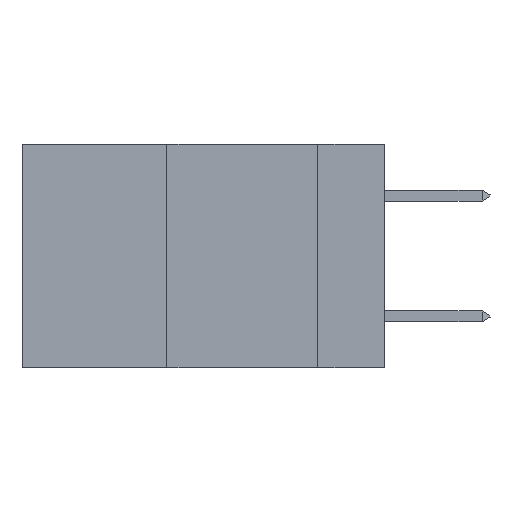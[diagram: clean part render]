
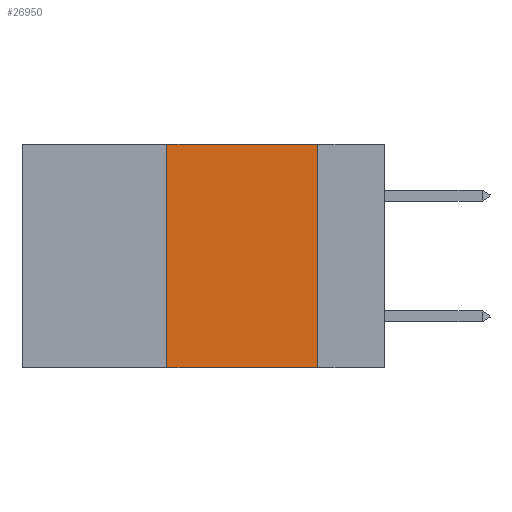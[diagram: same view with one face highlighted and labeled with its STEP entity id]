
A CAD part, left-side view. The second image highlights one B-rep face of the part: STEP entity #26950.
In plain terms, the highlighted planar face has unit normal (-1, 0, 0).
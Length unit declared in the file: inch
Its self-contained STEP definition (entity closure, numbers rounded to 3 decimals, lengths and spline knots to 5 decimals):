
#184 = VECTOR ( 'NONE', #4206, 39.37008 ) ;
#1067 = DIRECTION ( 'NONE',  ( 0., 0., -1. ) ) ;
#1257 = CARTESIAN_POINT ( 'NONE',  ( 0., 0.11, -0.37 ) ) ;
#2582 = CARTESIAN_POINT ( 'NONE',  ( 0., 0.6, -0.37 ) ) ;
#2880 = EDGE_LOOP ( 'NONE', ( #27715, #11392, #15418, #25714 ) ) ;
#3241 = CARTESIAN_POINT ( 'NONE',  ( 0., 0.6, 0. ) ) ;
#4206 = DIRECTION ( 'NONE',  ( 0., 0., 1. ) ) ;
#5151 = CARTESIAN_POINT ( 'NONE',  ( 0., 0.6, 0. ) ) ;
#6396 = VECTOR ( 'NONE', #27326, 39.37008 ) ;
#6772 = AXIS2_PLACEMENT_3D ( 'NONE', #3241, #17424, #1067 ) ;
#6932 = EDGE_CURVE ( 'NONE', #11074, #27075, #13192, .T. ) ;
#7243 = LINE ( 'NONE', #22990, #184 ) ;
#7800 = LINE ( 'NONE', #2582, #27742 ) ;
#9862 = VECTOR ( 'NONE', #24137, 39.37008 ) ;
#10455 = PLANE ( 'NONE',  #6772 ) ;
#10958 = CARTESIAN_POINT ( 'NONE',  ( 0., 0.11, 0. ) ) ;
#11074 = VERTEX_POINT ( 'NONE', #20526 ) ;
#11392 = ORIENTED_EDGE ( 'NONE', *, *, #6932, .F. ) ;
#12003 = EDGE_CURVE ( 'NONE', #27075, #12298, #18589, .T. ) ;
#12298 = VERTEX_POINT ( 'NONE', #1257 ) ;
#13192 = LINE ( 'NONE', #5151, #9862 ) ;
#15418 = ORIENTED_EDGE ( 'NONE', *, *, #27625, .F. ) ;
#17424 = DIRECTION ( 'NONE',  ( 1., 0., 0. ) ) ;
#17746 = CARTESIAN_POINT ( 'NONE',  ( 0., 0.11, 0. ) ) ;
#18307 = EDGE_CURVE ( 'NONE', #19309, #12298, #7800, .T. ) ;
#18589 = LINE ( 'NONE', #17746, #6396 ) ;
#19309 = VERTEX_POINT ( 'NONE', #25173 ) ;
#20526 = CARTESIAN_POINT ( 'NONE',  ( 0., 0.36, 0. ) ) ;
#22990 = CARTESIAN_POINT ( 'NONE',  ( 0., 0.36, 0. ) ) ;
#24137 = DIRECTION ( 'NONE',  ( 0., -1., 0. ) ) ;
#25173 = CARTESIAN_POINT ( 'NONE',  ( 0., 0.36, -0.37 ) ) ;
#25714 = ORIENTED_EDGE ( 'NONE', *, *, #18307, .T. ) ;
#26950 = ADVANCED_FACE ( 'NONE', ( #28000 ), #10455, .F. ) ;
#27075 = VERTEX_POINT ( 'NONE', #10958 ) ;
#27326 = DIRECTION ( 'NONE',  ( 0., 0., -1. ) ) ;
#27625 = EDGE_CURVE ( 'NONE', #19309, #11074, #7243, .T. ) ;
#27715 = ORIENTED_EDGE ( 'NONE', *, *, #12003, .F. ) ;
#27742 = VECTOR ( 'NONE', #28611, 39.37008 ) ;
#28000 = FACE_OUTER_BOUND ( 'NONE', #2880, .T. ) ;
#28611 = DIRECTION ( 'NONE',  ( 0., -1., 0. ) ) ;
